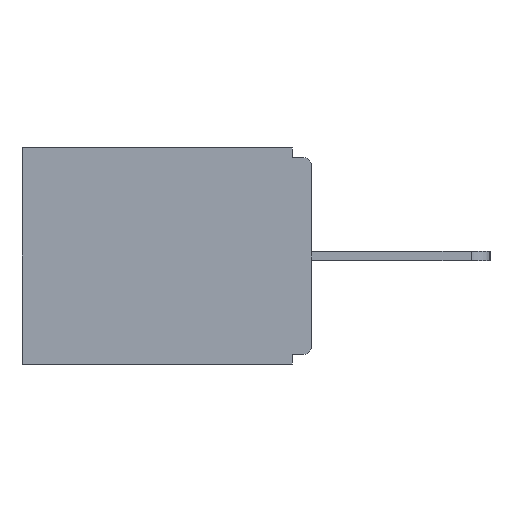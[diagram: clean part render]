
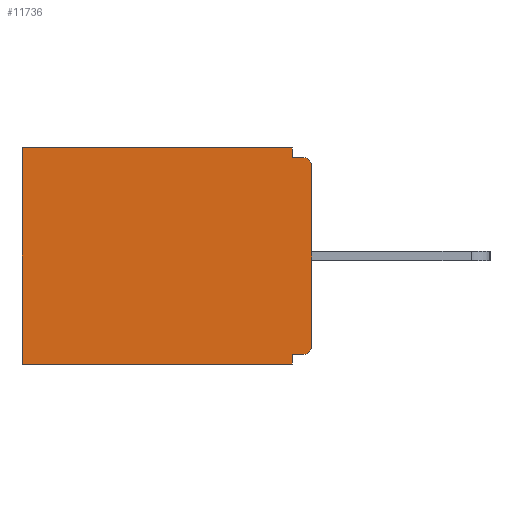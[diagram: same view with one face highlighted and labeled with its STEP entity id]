
A CAD part, left-side view. The second image highlights one B-rep face of the part: STEP entity #11736.
In plain terms, the highlighted planar face has unit normal (-1, 0, 0).
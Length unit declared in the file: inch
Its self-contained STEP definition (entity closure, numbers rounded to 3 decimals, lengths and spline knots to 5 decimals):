
#229 = CARTESIAN_POINT ( 'NONE',  ( 0.298, 0.015, -0.313 ) ) ;
#738 = VECTOR ( 'NONE', #3319, 39.37008 ) ;
#1029 = ORIENTED_EDGE ( 'NONE', *, *, #6496, .T. ) ;
#1217 = EDGE_CURVE ( 'NONE', #2076, #11894, #3130, .T. ) ;
#1272 = DIRECTION ( 'NONE',  ( 0., 0., -1. ) ) ;
#1287 = CARTESIAN_POINT ( 'NONE',  ( 0.298, 0., -0.343 ) ) ;
#1526 = VECTOR ( 'NONE', #10083, 39.37008 ) ;
#1793 = CARTESIAN_POINT ( 'NONE',  ( 0.298, 0., 0. ) ) ;
#1880 = CARTESIAN_POINT ( 'NONE',  ( 0.298, 0., -0.313 ) ) ;
#2076 = VERTEX_POINT ( 'NONE', #4550 ) ;
#2370 = CARTESIAN_POINT ( 'NONE',  ( 0.298, 0., -0.015 ) ) ;
#2490 = DIRECTION ( 'NONE',  ( 0., -1., 0. ) ) ;
#3076 = CARTESIAN_POINT ( 'NONE',  ( 0.298, 0., 0. ) ) ;
#3130 = LINE ( 'NONE', #2370, #8636 ) ;
#3319 = DIRECTION ( 'NONE',  ( 0., 1., 0. ) ) ;
#3476 = LINE ( 'NONE', #12281, #738 ) ;
#3535 = CARTESIAN_POINT ( 'NONE',  ( 0.298, 0.031, -0.343 ) ) ;
#3545 = ORIENTED_EDGE ( 'NONE', *, *, #12560, .T. ) ;
#3898 = EDGE_CURVE ( 'NONE', #11459, #8281, #10409, .T. ) ;
#3902 = DIRECTION ( 'NONE',  ( 1., 0., 0. ) ) ;
#4022 = VECTOR ( 'NONE', #4546, 39.37008 ) ;
#4378 = VECTOR ( 'NONE', #5677, 39.37008 ) ;
#4524 = ORIENTED_EDGE ( 'NONE', *, *, #10621, .T. ) ;
#4546 = DIRECTION ( 'NONE',  ( 0., 0., -1. ) ) ;
#4550 = CARTESIAN_POINT ( 'NONE',  ( 0.298, 0.031, -0.015 ) ) ;
#4675 = VERTEX_POINT ( 'NONE', #10891 ) ;
#4733 = AXIS2_PLACEMENT_3D ( 'NONE', #229, #7269, #1272 ) ;
#4961 = LINE ( 'NONE', #9264, #4022 ) ;
#4995 = EDGE_CURVE ( 'NONE', #4675, #9574, #6842, .T. ) ;
#5023 = VECTOR ( 'NONE', #8211, 39.37008 ) ;
#5280 = EDGE_CURVE ( 'NONE', #10561, #9663, #3476, .T. ) ;
#5337 = DIRECTION ( 'NONE',  ( 0., 1., 0. ) ) ;
#5383 = VECTOR ( 'NONE', #5337, 39.37008 ) ;
#5466 = CARTESIAN_POINT ( 'NONE',  ( 0.298, 0.015, -0.03 ) ) ;
#5470 = VERTEX_POINT ( 'NONE', #8524 ) ;
#5624 = ORIENTED_EDGE ( 'NONE', *, *, #9724, .F. ) ;
#5677 = DIRECTION ( 'NONE',  ( 0., 0., -1. ) ) ;
#5805 = VECTOR ( 'NONE', #12470, 39.37008 ) ;
#5965 = FACE_OUTER_BOUND ( 'NONE', #6923, .T. ) ;
#6151 = ORIENTED_EDGE ( 'NONE', *, *, #4995, .F. ) ;
#6420 = DIRECTION ( 'NONE',  ( 0., 0., -1. ) ) ;
#6496 = EDGE_CURVE ( 'NONE', #5470, #8487, #10634, .T. ) ;
#6842 = LINE ( 'NONE', #12238, #1526 ) ;
#6923 = EDGE_LOOP ( 'NONE', ( #9123, #9180, #10271, #1029, #3545, #9585, #5624, #9092, #4524, #6151 ) ) ;
#7127 = AXIS2_PLACEMENT_3D ( 'NONE', #5466, #12001, #6420 ) ;
#7269 = DIRECTION ( 'NONE',  ( -1., 0., 0. ) ) ;
#7555 = LINE ( 'NONE', #12211, #4378 ) ;
#7784 = PLANE ( 'NONE',  #12171 ) ;
#8047 = CARTESIAN_POINT ( 'NONE',  ( 0.298, 0.46, 0. ) ) ;
#8104 = LINE ( 'NONE', #9751, #5805 ) ;
#8211 = DIRECTION ( 'NONE',  ( 0., 1., 0. ) ) ;
#8281 = VERTEX_POINT ( 'NONE', #11213 ) ;
#8487 = VERTEX_POINT ( 'NONE', #8047 ) ;
#8514 = CARTESIAN_POINT ( 'NONE',  ( 0.298, 0.031, -0.328 ) ) ;
#8524 = CARTESIAN_POINT ( 'NONE',  ( 0.298, 0.031, 0. ) ) ;
#8636 = VECTOR ( 'NONE', #2490, 39.37008 ) ;
#9092 = ORIENTED_EDGE ( 'NONE', *, *, #5280, .F. ) ;
#9123 = ORIENTED_EDGE ( 'NONE', *, *, #10158, .T. ) ;
#9180 = ORIENTED_EDGE ( 'NONE', *, *, #1217, .F. ) ;
#9264 = CARTESIAN_POINT ( 'NONE',  ( 0.298, 0.031, -0.343 ) ) ;
#9574 = VERTEX_POINT ( 'NONE', #1880 ) ;
#9585 = ORIENTED_EDGE ( 'NONE', *, *, #3898, .F. ) ;
#9663 = VERTEX_POINT ( 'NONE', #8514 ) ;
#9724 = EDGE_CURVE ( 'NONE', #9663, #11459, #7555, .T. ) ;
#9751 = CARTESIAN_POINT ( 'NONE',  ( 0.298, 0.46, 0. ) ) ;
#10083 = DIRECTION ( 'NONE',  ( 0., 0., -1. ) ) ;
#10158 = EDGE_CURVE ( 'NONE', #4675, #11894, #11853, .T. ) ;
#10271 = ORIENTED_EDGE ( 'NONE', *, *, #10742, .F. ) ;
#10409 = LINE ( 'NONE', #1287, #5383 ) ;
#10558 = DIRECTION ( 'NONE',  ( 0., 0., -1. ) ) ;
#10561 = VERTEX_POINT ( 'NONE', #12510 ) ;
#10621 = EDGE_CURVE ( 'NONE', #10561, #9574, #12399, .T. ) ;
#10634 = LINE ( 'NONE', #3076, #5023 ) ;
#10742 = EDGE_CURVE ( 'NONE', #5470, #2076, #4961, .T. ) ;
#10891 = CARTESIAN_POINT ( 'NONE',  ( 0.298, 0., -0.03 ) ) ;
#11213 = CARTESIAN_POINT ( 'NONE',  ( 0.298, 0.46, -0.343 ) ) ;
#11459 = VERTEX_POINT ( 'NONE', #3535 ) ;
#11658 = CARTESIAN_POINT ( 'NONE',  ( 0.298, 0.015, -0.015 ) ) ;
#11736 = ADVANCED_FACE ( 'NONE', ( #5965 ), #7784, .F. ) ;
#11853 = CIRCLE ( 'NONE', #7127, 0.015 ) ;
#11894 = VERTEX_POINT ( 'NONE', #11658 ) ;
#12001 = DIRECTION ( 'NONE',  ( -1., 0., 0. ) ) ;
#12171 = AXIS2_PLACEMENT_3D ( 'NONE', #1793, #3902, #10558 ) ;
#12211 = CARTESIAN_POINT ( 'NONE',  ( 0.298, 0.031, -0.343 ) ) ;
#12238 = CARTESIAN_POINT ( 'NONE',  ( 0.298, 0., 0. ) ) ;
#12281 = CARTESIAN_POINT ( 'NONE',  ( 0.298, 0., -0.328 ) ) ;
#12399 = CIRCLE ( 'NONE', #4733, 0.015 ) ;
#12470 = DIRECTION ( 'NONE',  ( 0., 0., -1. ) ) ;
#12510 = CARTESIAN_POINT ( 'NONE',  ( 0.298, 0.015, -0.328 ) ) ;
#12560 = EDGE_CURVE ( 'NONE', #8487, #8281, #8104, .T. ) ;
